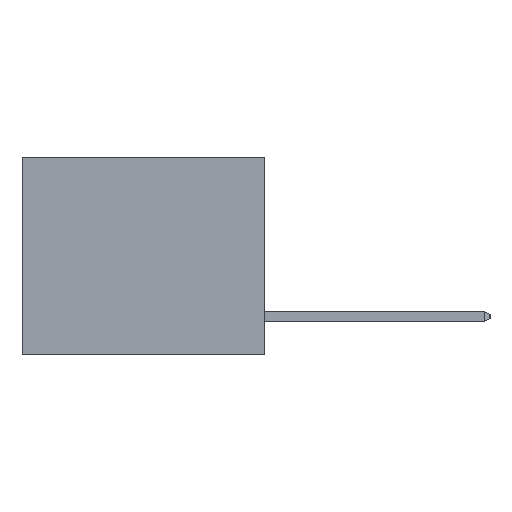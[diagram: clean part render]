
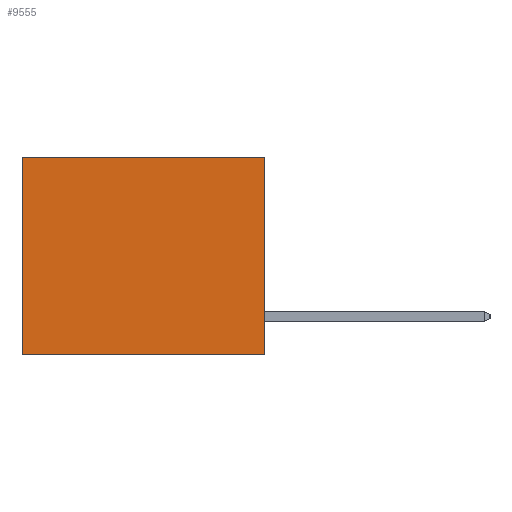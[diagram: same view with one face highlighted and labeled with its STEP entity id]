
A CAD part, left-side view. The second image highlights one B-rep face of the part: STEP entity #9555.
In plain terms, the highlighted planar face has unit normal (-1, 0, 0).
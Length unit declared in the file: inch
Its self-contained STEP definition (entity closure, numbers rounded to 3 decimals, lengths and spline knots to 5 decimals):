
#4 = VECTOR ( 'NONE', #344, 39.37008 ) ;
#344 = DIRECTION ( 'NONE',  ( 0., 0., -1. ) ) ;
#446 = ORIENTED_EDGE ( 'NONE', *, *, #12458, .F. ) ;
#1076 = VERTEX_POINT ( 'NONE', #20860 ) ;
#2595 = VECTOR ( 'NONE', #14794, 39.37008 ) ;
#2637 = PLANE ( 'NONE',  #23921 ) ;
#4025 = DIRECTION ( 'NONE',  ( 0., 1., 0. ) ) ;
#7334 = VERTEX_POINT ( 'NONE', #23800 ) ;
#7983 = CARTESIAN_POINT ( 'NONE',  ( 0.3165, 0., -0.49 ) ) ;
#8056 = EDGE_LOOP ( 'NONE', ( #23601, #8204, #446, #21456 ) ) ;
#8095 = CARTESIAN_POINT ( 'NONE',  ( 0.3165, 0., -0.49 ) ) ;
#8204 = ORIENTED_EDGE ( 'NONE', *, *, #14857, .F. ) ;
#8522 = LINE ( 'NONE', #11260, #2595 ) ;
#8574 = LINE ( 'NONE', #15381, #14213 ) ;
#9555 = ADVANCED_FACE ( 'NONE', ( #19346 ), #2637, .F. ) ;
#11260 = CARTESIAN_POINT ( 'NONE',  ( 0.3165, 0.6, -0.49 ) ) ;
#11275 = VERTEX_POINT ( 'NONE', #18665 ) ;
#12458 = EDGE_CURVE ( 'NONE', #16178, #1076, #20100, .T. ) ;
#12714 = EDGE_CURVE ( 'NONE', #7334, #11275, #8522, .T. ) ;
#14213 = VECTOR ( 'NONE', #4025, 39.37008 ) ;
#14794 = DIRECTION ( 'NONE',  ( 0., 0., -1. ) ) ;
#14857 = EDGE_CURVE ( 'NONE', #1076, #11275, #8574, .T. ) ;
#15381 = CARTESIAN_POINT ( 'NONE',  ( 0.3165, 0., -0.49 ) ) ;
#16092 = VECTOR ( 'NONE', #16690, 39.37008 ) ;
#16178 = VERTEX_POINT ( 'NONE', #23447 ) ;
#16672 = LINE ( 'NONE', #22348, #16092 ) ;
#16690 = DIRECTION ( 'NONE',  ( 0., 1., 0. ) ) ;
#18665 = CARTESIAN_POINT ( 'NONE',  ( 0.3165, 0.6, -0.49 ) ) ;
#19346 = FACE_OUTER_BOUND ( 'NONE', #8056, .T. ) ;
#20100 = LINE ( 'NONE', #7983, #4 ) ;
#20860 = CARTESIAN_POINT ( 'NONE',  ( 0.3165, 0., -0.49 ) ) ;
#21456 = ORIENTED_EDGE ( 'NONE', *, *, #23825, .T. ) ;
#22348 = CARTESIAN_POINT ( 'NONE',  ( 0.3165, 0., 0. ) ) ;
#23249 = DIRECTION ( 'NONE',  ( 0., 0., -1. ) ) ;
#23324 = DIRECTION ( 'NONE',  ( 1., 0., 0. ) ) ;
#23447 = CARTESIAN_POINT ( 'NONE',  ( 0.3165, 0., 0. ) ) ;
#23601 = ORIENTED_EDGE ( 'NONE', *, *, #12714, .T. ) ;
#23800 = CARTESIAN_POINT ( 'NONE',  ( 0.3165, 0.6, 0. ) ) ;
#23825 = EDGE_CURVE ( 'NONE', #16178, #7334, #16672, .T. ) ;
#23921 = AXIS2_PLACEMENT_3D ( 'NONE', #8095, #23324, #23249 ) ;
